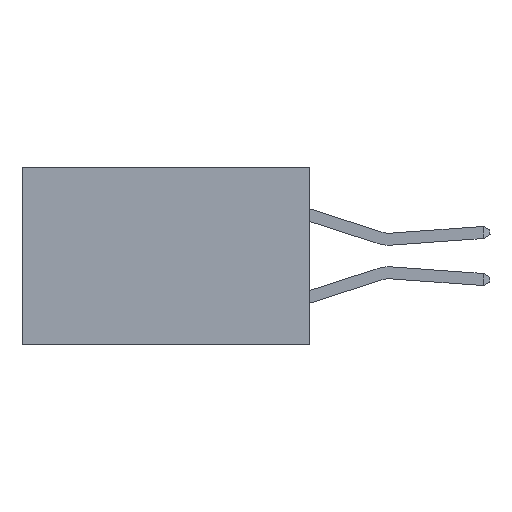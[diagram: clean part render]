
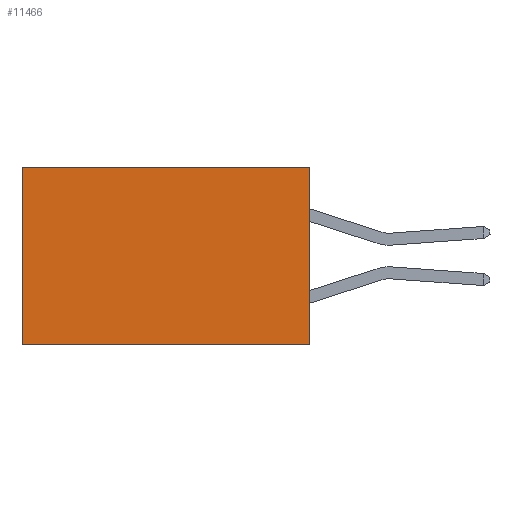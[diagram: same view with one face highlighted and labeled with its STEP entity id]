
A CAD part, left-side view. The second image highlights one B-rep face of the part: STEP entity #11466.
In plain terms, the highlighted planar face has unit normal (-1, 0, 0).
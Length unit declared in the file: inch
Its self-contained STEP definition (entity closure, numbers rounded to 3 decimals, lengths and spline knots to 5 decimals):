
#76 = CARTESIAN_POINT ( 'NONE',  ( 0.2615, 0., 0. ) ) ;
#463 = DIRECTION ( 'NONE',  ( 0., 1., 0. ) ) ;
#1178 = LINE ( 'NONE', #11284, #7261 ) ;
#1236 = ORIENTED_EDGE ( 'NONE', *, *, #5818, .F. ) ;
#1760 = CARTESIAN_POINT ( 'NONE',  ( 0.2615, 0.6, -0.37 ) ) ;
#1832 = VERTEX_POINT ( 'NONE', #9951 ) ;
#2465 = DIRECTION ( 'NONE',  ( 0., 0., -1. ) ) ;
#2493 = DIRECTION ( 'NONE',  ( 1., 0., 0. ) ) ;
#2586 = CARTESIAN_POINT ( 'NONE',  ( 0.2615, 0., -0.37 ) ) ;
#2768 = PLANE ( 'NONE',  #12175 ) ;
#2899 = CARTESIAN_POINT ( 'NONE',  ( 0.2615, 0.6, 0. ) ) ;
#3040 = VECTOR ( 'NONE', #463, 39.37008 ) ;
#4125 = DIRECTION ( 'NONE',  ( 0., 1., 0. ) ) ;
#4439 = CARTESIAN_POINT ( 'NONE',  ( 0.2615, 0., -0.37 ) ) ;
#5818 = EDGE_CURVE ( 'NONE', #10042, #1832, #10461, .T. ) ;
#5832 = EDGE_CURVE ( 'NONE', #9262, #10299, #1178, .T. ) ;
#7261 = VECTOR ( 'NONE', #11033, 39.37008 ) ;
#7958 = VECTOR ( 'NONE', #11691, 39.37008 ) ;
#8302 = LINE ( 'NONE', #4439, #13592 ) ;
#9262 = VERTEX_POINT ( 'NONE', #2899 ) ;
#9473 = EDGE_CURVE ( 'NONE', #10042, #9262, #12396, .T. ) ;
#9911 = ORIENTED_EDGE ( 'NONE', *, *, #13067, .F. ) ;
#9951 = CARTESIAN_POINT ( 'NONE',  ( 0.2615, 0., -0.37 ) ) ;
#10042 = VERTEX_POINT ( 'NONE', #11013 ) ;
#10160 = FACE_OUTER_BOUND ( 'NONE', #14238, .T. ) ;
#10299 = VERTEX_POINT ( 'NONE', #1760 ) ;
#10461 = LINE ( 'NONE', #11715, #7958 ) ;
#11013 = CARTESIAN_POINT ( 'NONE',  ( 0.2615, 0., 0. ) ) ;
#11033 = DIRECTION ( 'NONE',  ( 0., 0., -1. ) ) ;
#11284 = CARTESIAN_POINT ( 'NONE',  ( 0.2615, 0.6, -0.37 ) ) ;
#11466 = ADVANCED_FACE ( 'NONE', ( #10160 ), #2768, .F. ) ;
#11691 = DIRECTION ( 'NONE',  ( 0., 0., -1. ) ) ;
#11715 = CARTESIAN_POINT ( 'NONE',  ( 0.2615, 0., -0.37 ) ) ;
#12175 = AXIS2_PLACEMENT_3D ( 'NONE', #2586, #2493, #2465 ) ;
#12396 = LINE ( 'NONE', #76, #3040 ) ;
#12404 = ORIENTED_EDGE ( 'NONE', *, *, #5832, .T. ) ;
#13067 = EDGE_CURVE ( 'NONE', #1832, #10299, #8302, .T. ) ;
#13592 = VECTOR ( 'NONE', #4125, 39.37008 ) ;
#13717 = ORIENTED_EDGE ( 'NONE', *, *, #9473, .T. ) ;
#14238 = EDGE_LOOP ( 'NONE', ( #12404, #9911, #1236, #13717 ) ) ;
